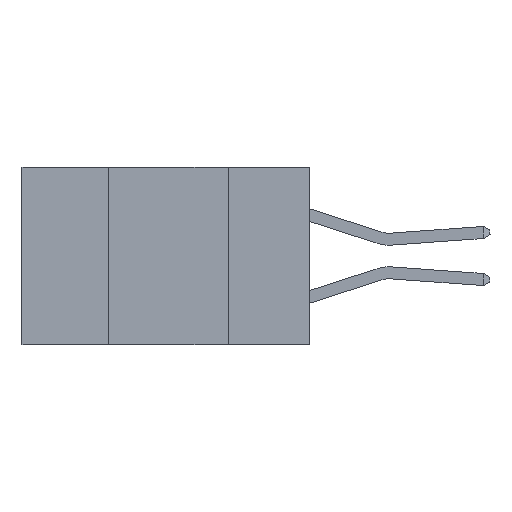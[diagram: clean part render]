
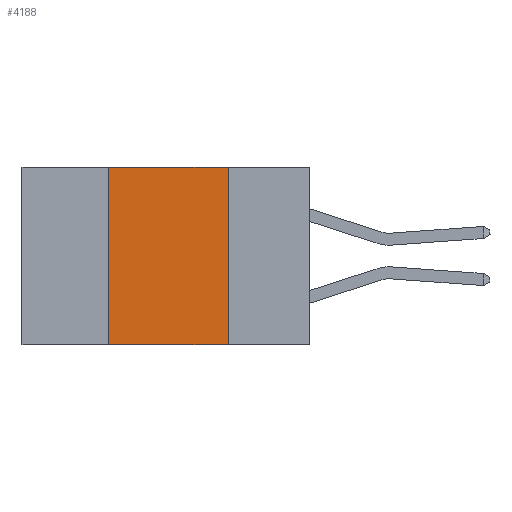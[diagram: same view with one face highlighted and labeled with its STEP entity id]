
A CAD part, left-side view. The second image highlights one B-rep face of the part: STEP entity #4188.
In plain terms, the highlighted planar face has unit normal (-1, 0, 0).
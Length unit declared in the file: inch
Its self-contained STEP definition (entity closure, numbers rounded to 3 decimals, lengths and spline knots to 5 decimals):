
#1236 = CARTESIAN_POINT ( 'NONE',  ( 0., 0.6, 0. ) ) ;
#2558 = ORIENTED_EDGE ( 'NONE', *, *, #18549, .F. ) ;
#3041 = PLANE ( 'NONE',  #18450 ) ;
#3087 = LINE ( 'NONE', #18652, #15563 ) ;
#3506 = VERTEX_POINT ( 'NONE', #5239 ) ;
#3596 = CARTESIAN_POINT ( 'NONE',  ( 0., 0.6, -0.37 ) ) ;
#3914 = ORIENTED_EDGE ( 'NONE', *, *, #17157, .T. ) ;
#3960 = CARTESIAN_POINT ( 'NONE',  ( 0., 0.17, -0.37 ) ) ;
#4188 = ADVANCED_FACE ( 'NONE', ( #18063 ), #3041, .F. ) ;
#4584 = DIRECTION ( 'NONE',  ( 0., -1., 0. ) ) ;
#4816 = VERTEX_POINT ( 'NONE', #20084 ) ;
#5239 = CARTESIAN_POINT ( 'NONE',  ( 0., 0.17, 0. ) ) ;
#5693 = LINE ( 'NONE', #1236, #6438 ) ;
#6384 = EDGE_LOOP ( 'NONE', ( #2558, #13841, #12557, #3914 ) ) ;
#6438 = VECTOR ( 'NONE', #4584, 39.37008 ) ;
#6932 = CARTESIAN_POINT ( 'NONE',  ( 0., 0.42, -0.37 ) ) ;
#6980 = VERTEX_POINT ( 'NONE', #3960 ) ;
#7589 = CARTESIAN_POINT ( 'NONE',  ( 0., 0.6, 0. ) ) ;
#7606 = EDGE_CURVE ( 'NONE', #4816, #3506, #5693, .T. ) ;
#7971 = EDGE_CURVE ( 'NONE', #8629, #4816, #3087, .T. ) ;
#8629 = VERTEX_POINT ( 'NONE', #6932 ) ;
#9496 = DIRECTION ( 'NONE',  ( 0., 0., -1. ) ) ;
#11695 = DIRECTION ( 'NONE',  ( 0., -1., 0. ) ) ;
#12557 = ORIENTED_EDGE ( 'NONE', *, *, #7971, .F. ) ;
#12726 = DIRECTION ( 'NONE',  ( 0., 0., -1. ) ) ;
#13841 = ORIENTED_EDGE ( 'NONE', *, *, #7606, .F. ) ;
#13851 = CARTESIAN_POINT ( 'NONE',  ( 0., 0.17, 0. ) ) ;
#15563 = VECTOR ( 'NONE', #19267, 39.37008 ) ;
#16800 = VECTOR ( 'NONE', #11695, 39.37008 ) ;
#17157 = EDGE_CURVE ( 'NONE', #8629, #6980, #19879, .T. ) ;
#18063 = FACE_OUTER_BOUND ( 'NONE', #6384, .T. ) ;
#18450 = AXIS2_PLACEMENT_3D ( 'NONE', #7589, #18995, #12726 ) ;
#18549 = EDGE_CURVE ( 'NONE', #3506, #6980, #19290, .T. ) ;
#18652 = CARTESIAN_POINT ( 'NONE',  ( 0., 0.42, 0. ) ) ;
#18995 = DIRECTION ( 'NONE',  ( 1., 0., 0. ) ) ;
#19042 = VECTOR ( 'NONE', #9496, 39.37008 ) ;
#19267 = DIRECTION ( 'NONE',  ( 0., 0., 1. ) ) ;
#19290 = LINE ( 'NONE', #13851, #19042 ) ;
#19879 = LINE ( 'NONE', #3596, #16800 ) ;
#20084 = CARTESIAN_POINT ( 'NONE',  ( 0., 0.42, 0. ) ) ;
